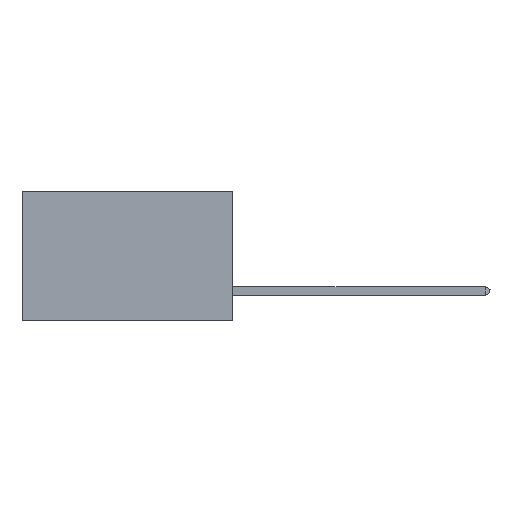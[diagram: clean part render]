
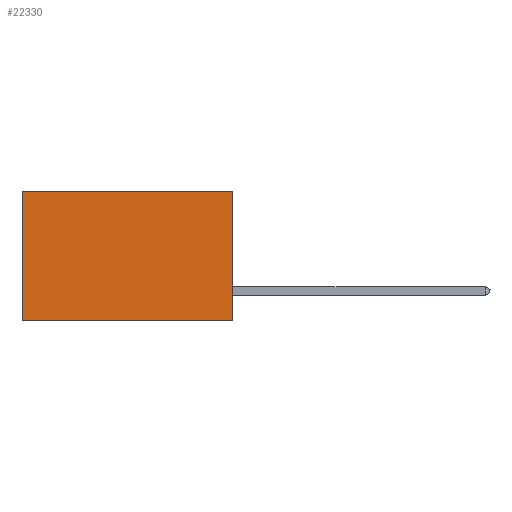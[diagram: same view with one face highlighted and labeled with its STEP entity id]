
A CAD part, left-side view. The second image highlights one B-rep face of the part: STEP entity #22330.
In plain terms, the highlighted planar face has unit normal (-1, 0, 0).
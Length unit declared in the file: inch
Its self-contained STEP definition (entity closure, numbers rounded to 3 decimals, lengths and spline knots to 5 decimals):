
#1032 = CARTESIAN_POINT ( 'NONE',  ( 0.2875, 0.6, 0. ) ) ;
#1185 = ORIENTED_EDGE ( 'NONE', *, *, #21048, .T. ) ;
#1211 = ORIENTED_EDGE ( 'NONE', *, *, #18521, .T. ) ;
#1452 = PLANE ( 'NONE',  #13138 ) ;
#1587 = EDGE_LOOP ( 'NONE', ( #1211, #4589, #24071, #1185 ) ) ;
#2168 = VERTEX_POINT ( 'NONE', #23467 ) ;
#4589 = ORIENTED_EDGE ( 'NONE', *, *, #27613, .F. ) ;
#4617 = LINE ( 'NONE', #10604, #14387 ) ;
#5632 = DIRECTION ( 'NONE',  ( 0., 0., -1. ) ) ;
#6423 = LINE ( 'NONE', #25515, #18320 ) ;
#6576 = EDGE_CURVE ( 'NONE', #2168, #10740, #19822, .T. ) ;
#7111 = CARTESIAN_POINT ( 'NONE',  ( 0.2875, 0., -0.37 ) ) ;
#8005 = VECTOR ( 'NONE', #27719, 39.37008 ) ;
#8515 = DIRECTION ( 'NONE',  ( 1., 0., 0. ) ) ;
#8821 = DIRECTION ( 'NONE',  ( 0., 0., -1. ) ) ;
#10090 = CARTESIAN_POINT ( 'NONE',  ( 0.2875, 0., -0.37 ) ) ;
#10604 = CARTESIAN_POINT ( 'NONE',  ( 0.2875, 0.6, 0. ) ) ;
#10740 = VERTEX_POINT ( 'NONE', #10090 ) ;
#11432 = VERTEX_POINT ( 'NONE', #1032 ) ;
#11611 = LINE ( 'NONE', #7111, #8005 ) ;
#12387 = VERTEX_POINT ( 'NONE', #14218 ) ;
#13138 = AXIS2_PLACEMENT_3D ( 'NONE', #20193, #8515, #27057 ) ;
#13684 = VECTOR ( 'NONE', #8821, 39.37008 ) ;
#14218 = CARTESIAN_POINT ( 'NONE',  ( 0.2875, 0.6, -0.37 ) ) ;
#14387 = VECTOR ( 'NONE', #5632, 39.37008 ) ;
#17508 = DIRECTION ( 'NONE',  ( 0., 1., 0. ) ) ;
#18320 = VECTOR ( 'NONE', #17508, 39.37008 ) ;
#18521 = EDGE_CURVE ( 'NONE', #11432, #12387, #4617, .T. ) ;
#19822 = LINE ( 'NONE', #20206, #13684 ) ;
#20193 = CARTESIAN_POINT ( 'NONE',  ( 0.2875, 0., 0. ) ) ;
#20206 = CARTESIAN_POINT ( 'NONE',  ( 0.2875, 0., 0. ) ) ;
#21048 = EDGE_CURVE ( 'NONE', #2168, #11432, #6423, .T. ) ;
#22330 = ADVANCED_FACE ( 'NONE', ( #27263 ), #1452, .F. ) ;
#23467 = CARTESIAN_POINT ( 'NONE',  ( 0.2875, 0., 0. ) ) ;
#24071 = ORIENTED_EDGE ( 'NONE', *, *, #6576, .F. ) ;
#25515 = CARTESIAN_POINT ( 'NONE',  ( 0.2875, 0., 0. ) ) ;
#27057 = DIRECTION ( 'NONE',  ( 0., 0., -1. ) ) ;
#27263 = FACE_OUTER_BOUND ( 'NONE', #1587, .T. ) ;
#27613 = EDGE_CURVE ( 'NONE', #10740, #12387, #11611, .T. ) ;
#27719 = DIRECTION ( 'NONE',  ( 0., 1., 0. ) ) ;
